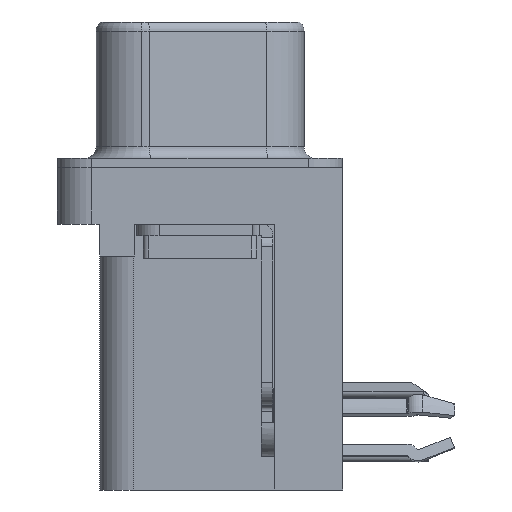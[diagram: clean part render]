
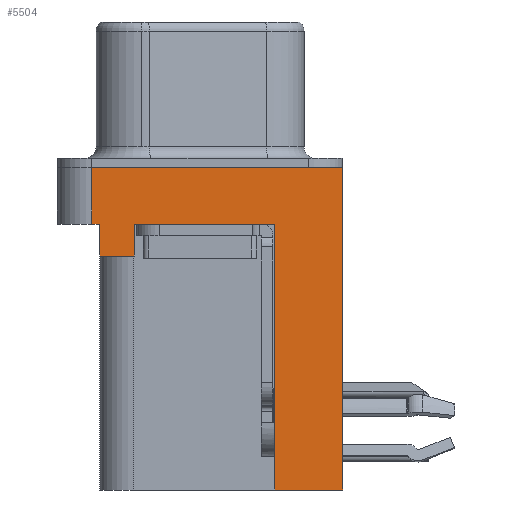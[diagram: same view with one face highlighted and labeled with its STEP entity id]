
A CAD part, left-side view. The second image highlights one B-rep face of the part: STEP entity #5504.
In plain terms, the highlighted planar face has unit normal (-1, 0, 0).
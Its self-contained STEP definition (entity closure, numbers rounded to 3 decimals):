
#59 = DIRECTION ( 'NONE',  ( 0., 0., 1. ) ) ;
#558 = DIRECTION ( 'NONE',  ( 0., 1., 0. ) ) ;
#563 = LINE ( 'NONE', #5693, #10229 ) ;
#747 = DIRECTION ( 'NONE',  ( 0., 0., 1. ) ) ;
#911 = LINE ( 'NONE', #16725, #11830 ) ;
#998 = EDGE_CURVE ( 'NONE', #13759, #1258, #18729, .T. ) ;
#1258 = VERTEX_POINT ( 'NONE', #9935 ) ;
#1273 = VERTEX_POINT ( 'NONE', #5221 ) ;
#1402 = EDGE_LOOP ( 'NONE', ( #3273, #16153, #15935, #18890, #13981, #10884, #10069, #7469, #7784, #3710 ) ) ;
#1704 = CARTESIAN_POINT ( 'NONE',  ( -2.935, 2.895, -3.9 ) ) ;
#2537 = CARTESIAN_POINT ( 'NONE',  ( -2.935, 4.775, -2.5 ) ) ;
#3089 = EDGE_CURVE ( 'NONE', #9601, #19516, #4908, .T. ) ;
#3273 = ORIENTED_EDGE ( 'NONE', *, *, #998, .F. ) ;
#3677 = CARTESIAN_POINT ( 'NONE',  ( -2.935, -6.275, -2.5 ) ) ;
#3710 = ORIENTED_EDGE ( 'NONE', *, *, #14448, .T. ) ;
#4908 = LINE ( 'NONE', #11609, #5900 ) ;
#4963 = LINE ( 'NONE', #20684, #12829 ) ;
#5221 = CARTESIAN_POINT ( 'NONE',  ( -2.935, 2.895, -2.5 ) ) ;
#5504 = ADVANCED_FACE ( 'NONE', ( #20530 ), #6176, .T. ) ;
#5693 = CARTESIAN_POINT ( 'NONE',  ( -2.935, 4.425, -3.9 ) ) ;
#5818 = CARTESIAN_POINT ( 'NONE',  ( -2.935, 4.425, -3.9 ) ) ;
#5900 = VECTOR ( 'NONE', #8462, 1000. ) ;
#5906 = CARTESIAN_POINT ( 'NONE',  ( -2.935, -3.295, -14.2 ) ) ;
#6057 = CARTESIAN_POINT ( 'NONE',  ( -2.935, -6.275, 0. ) ) ;
#6176 = PLANE ( 'NONE',  #9117 ) ;
#6323 = DIRECTION ( 'NONE',  ( 0., -1., 0. ) ) ;
#6354 = LINE ( 'NONE', #7936, #6790 ) ;
#6790 = VECTOR ( 'NONE', #9507, 1000. ) ;
#7469 = ORIENTED_EDGE ( 'NONE', *, *, #8748, .F. ) ;
#7555 = VERTEX_POINT ( 'NONE', #2537 ) ;
#7784 = ORIENTED_EDGE ( 'NONE', *, *, #3089, .F. ) ;
#7936 = CARTESIAN_POINT ( 'NONE',  ( -2.935, 4.775, -2.5 ) ) ;
#8039 = LINE ( 'NONE', #19258, #8134 ) ;
#8134 = VECTOR ( 'NONE', #59, 1000. ) ;
#8394 = DIRECTION ( 'NONE',  ( 0., 0., 1. ) ) ;
#8462 = DIRECTION ( 'NONE',  ( 0., 1., 0. ) ) ;
#8524 = CARTESIAN_POINT ( 'NONE',  ( -2.935, -3.295, -14.2 ) ) ;
#8748 = EDGE_CURVE ( 'NONE', #19516, #13144, #16574, .T. ) ;
#9117 = AXIS2_PLACEMENT_3D ( 'NONE', #18949, #11000, #20735 ) ;
#9507 = DIRECTION ( 'NONE',  ( 0., 0., 1. ) ) ;
#9601 = VERTEX_POINT ( 'NONE', #19996 ) ;
#9647 = EDGE_CURVE ( 'NONE', #7555, #19603, #911, .T. ) ;
#9730 = VERTEX_POINT ( 'NONE', #1704 ) ;
#9775 = EDGE_CURVE ( 'NONE', #1273, #13144, #4963, .T. ) ;
#9935 = CARTESIAN_POINT ( 'NONE',  ( -2.935, -6.275, 0. ) ) ;
#9990 = LINE ( 'NONE', #14903, #16638 ) ;
#10069 = ORIENTED_EDGE ( 'NONE', *, *, #9775, .T. ) ;
#10229 = VECTOR ( 'NONE', #13561, 1000. ) ;
#10716 = VECTOR ( 'NONE', #20521, 1000. ) ;
#10884 = ORIENTED_EDGE ( 'NONE', *, *, #10904, .T. ) ;
#10904 = EDGE_CURVE ( 'NONE', #9730, #1273, #8039, .T. ) ;
#11000 = DIRECTION ( 'NONE',  ( -1., 0., 0. ) ) ;
#11513 = VECTOR ( 'NONE', #747, 1000. ) ;
#11609 = CARTESIAN_POINT ( 'NONE',  ( -2.935, -3.295, -14.2 ) ) ;
#11830 = VECTOR ( 'NONE', #15369, 1000. ) ;
#12205 = VERTEX_POINT ( 'NONE', #5818 ) ;
#12829 = VECTOR ( 'NONE', #6323, 1000. ) ;
#13144 = VERTEX_POINT ( 'NONE', #16081 ) ;
#13532 = LINE ( 'NONE', #3677, #17211 ) ;
#13561 = DIRECTION ( 'NONE',  ( 0., 0., 1. ) ) ;
#13609 = CARTESIAN_POINT ( 'NONE',  ( -2.935, 4.775, 0. ) ) ;
#13759 = VERTEX_POINT ( 'NONE', #13609 ) ;
#13981 = ORIENTED_EDGE ( 'NONE', *, *, #17570, .F. ) ;
#14448 = EDGE_CURVE ( 'NONE', #9601, #1258, #13532, .T. ) ;
#14903 = CARTESIAN_POINT ( 'NONE',  ( -2.935, 4.425, -3.9 ) ) ;
#15369 = DIRECTION ( 'NONE',  ( 0., -1., 0. ) ) ;
#15935 = ORIENTED_EDGE ( 'NONE', *, *, #9647, .T. ) ;
#16012 = EDGE_CURVE ( 'NONE', #12205, #19603, #563, .T. ) ;
#16081 = CARTESIAN_POINT ( 'NONE',  ( -2.935, -3.295, -2.5 ) ) ;
#16153 = ORIENTED_EDGE ( 'NONE', *, *, #20357, .F. ) ;
#16574 = LINE ( 'NONE', #8524, #11513 ) ;
#16638 = VECTOR ( 'NONE', #558, 1000. ) ;
#16725 = CARTESIAN_POINT ( 'NONE',  ( -2.935, -6.275, -2.5 ) ) ;
#17211 = VECTOR ( 'NONE', #8394, 1000. ) ;
#17570 = EDGE_CURVE ( 'NONE', #9730, #12205, #9990, .T. ) ;
#18729 = LINE ( 'NONE', #6057, #10716 ) ;
#18890 = ORIENTED_EDGE ( 'NONE', *, *, #16012, .F. ) ;
#18949 = CARTESIAN_POINT ( 'NONE',  ( -2.935, -6.275, -2.5 ) ) ;
#19258 = CARTESIAN_POINT ( 'NONE',  ( -2.935, 2.895, -3.9 ) ) ;
#19516 = VERTEX_POINT ( 'NONE', #5906 ) ;
#19603 = VERTEX_POINT ( 'NONE', #20566 ) ;
#19996 = CARTESIAN_POINT ( 'NONE',  ( -2.935, -6.275, -14.2 ) ) ;
#20357 = EDGE_CURVE ( 'NONE', #7555, #13759, #6354, .T. ) ;
#20521 = DIRECTION ( 'NONE',  ( 0., -1., 0. ) ) ;
#20530 = FACE_OUTER_BOUND ( 'NONE', #1402, .T. ) ;
#20566 = CARTESIAN_POINT ( 'NONE',  ( -2.935, 4.425, -2.5 ) ) ;
#20684 = CARTESIAN_POINT ( 'NONE',  ( -2.935, -6.275, -2.5 ) ) ;
#20735 = DIRECTION ( 'NONE',  ( 0., 0., 1. ) ) ;
